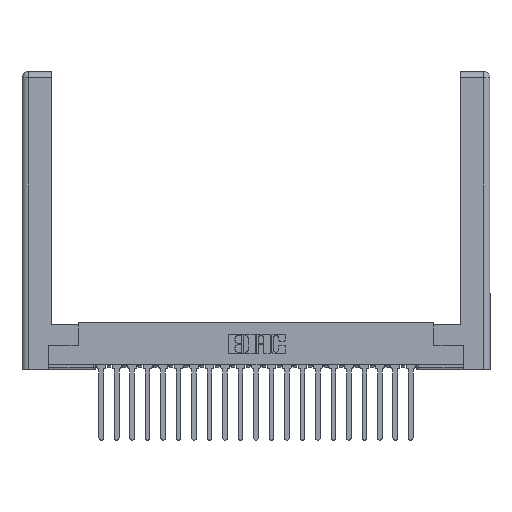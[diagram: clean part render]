
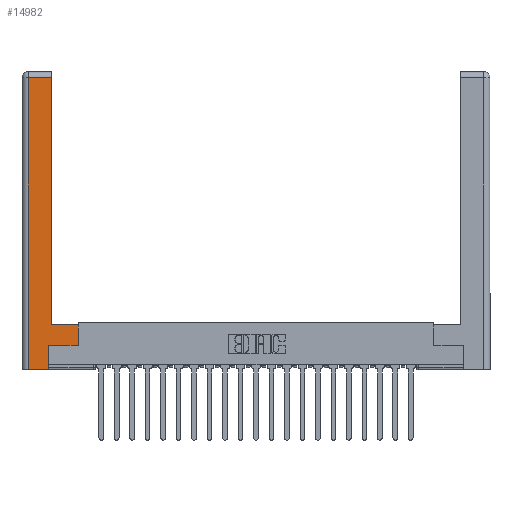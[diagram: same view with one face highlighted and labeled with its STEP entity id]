
A CAD part, top view. The second image highlights one B-rep face of the part: STEP entity #14982.
In plain terms, the highlighted planar face has unit normal (0, 0, 1).
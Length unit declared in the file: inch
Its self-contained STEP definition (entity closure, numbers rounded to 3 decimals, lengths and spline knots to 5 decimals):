
#617 = CARTESIAN_POINT ( 'NONE',  ( 0.0615, 2.94, 0. ) ) ;
#858 = PLANE ( 'NONE',  #6192 ) ;
#1038 = DIRECTION ( 'NONE',  ( 0., 1., 0. ) ) ;
#1102 = VERTEX_POINT ( 'NONE', #7507 ) ;
#2020 = CARTESIAN_POINT ( 'NONE',  ( 0.0615, 2.94, 0. ) ) ;
#2533 = VECTOR ( 'NONE', #12860, 39.37008 ) ;
#2578 = DIRECTION ( 'NONE',  ( 0., 1., 0. ) ) ;
#2597 = CARTESIAN_POINT ( 'NONE',  ( 0., 0., 0. ) ) ;
#2929 = FACE_OUTER_BOUND ( 'NONE', #4494, .T. ) ;
#3064 = EDGE_CURVE ( 'NONE', #12046, #16236, #20750, .T. ) ;
#3332 = EDGE_CURVE ( 'NONE', #23174, #12046, #17524, .T. ) ;
#3719 = ORIENTED_EDGE ( 'NONE', *, *, #6815, .T. ) ;
#3980 = ORIENTED_EDGE ( 'NONE', *, *, #19150, .T. ) ;
#4494 = EDGE_LOOP ( 'NONE', ( #23071, #3719, #3980, #4528, #10552, #19849, #20191, #16464 ) ) ;
#4528 = ORIENTED_EDGE ( 'NONE', *, *, #7918, .T. ) ;
#6113 = CARTESIAN_POINT ( 'NONE',  ( 0.295, 3., 0. ) ) ;
#6173 = LINE ( 'NONE', #617, #2533 ) ;
#6192 = AXIS2_PLACEMENT_3D ( 'NONE', #2597, #22149, #8065 ) ;
#6324 = CARTESIAN_POINT ( 'NONE',  ( 0.565, 0.245, 0. ) ) ;
#6553 = DIRECTION ( 'NONE',  ( 0., -1., 0. ) ) ;
#6815 = EDGE_CURVE ( 'NONE', #16236, #9266, #6173, .T. ) ;
#7507 = CARTESIAN_POINT ( 'NONE',  ( 0.265, 0., 0. ) ) ;
#7607 = VERTEX_POINT ( 'NONE', #6324 ) ;
#7918 = EDGE_CURVE ( 'NONE', #12849, #1102, #9459, .T. ) ;
#8065 = DIRECTION ( 'NONE',  ( -1., 0., 0. ) ) ;
#9266 = VERTEX_POINT ( 'NONE', #2020 ) ;
#9459 = LINE ( 'NONE', #15742, #12246 ) ;
#10511 = VECTOR ( 'NONE', #20896, 39.37008 ) ;
#10552 = ORIENTED_EDGE ( 'NONE', *, *, #19860, .T. ) ;
#11117 = DIRECTION ( 'NONE',  ( 0., 1., 0. ) ) ;
#11160 = EDGE_CURVE ( 'NONE', #7607, #23174, #21858, .T. ) ;
#11485 = VECTOR ( 'NONE', #1038, 39.37008 ) ;
#11532 = VECTOR ( 'NONE', #11117, 39.37008 ) ;
#11841 = LINE ( 'NONE', #11936, #18846 ) ;
#11936 = CARTESIAN_POINT ( 'NONE',  ( 0.0615, 0., 0. ) ) ;
#12046 = VERTEX_POINT ( 'NONE', #19767 ) ;
#12246 = VECTOR ( 'NONE', #12384, 39.37008 ) ;
#12384 = DIRECTION ( 'NONE',  ( 1., 0., 0. ) ) ;
#12849 = VERTEX_POINT ( 'NONE', #20310 ) ;
#12860 = DIRECTION ( 'NONE',  ( -1., 0., 0. ) ) ;
#13403 = VERTEX_POINT ( 'NONE', #16669 ) ;
#14428 = VECTOR ( 'NONE', #14737, 39.37008 ) ;
#14615 = LINE ( 'NONE', #17183, #18270 ) ;
#14737 = DIRECTION ( 'NONE',  ( 1., 0., 0. ) ) ;
#14982 = ADVANCED_FACE ( 'NONE', ( #2929 ), #858, .F. ) ;
#15058 = CARTESIAN_POINT ( 'NONE',  ( 0.295, 2.94, 0. ) ) ;
#15742 = CARTESIAN_POINT ( 'NONE',  ( 0.265, 0., 0. ) ) ;
#16236 = VERTEX_POINT ( 'NONE', #15058 ) ;
#16464 = ORIENTED_EDGE ( 'NONE', *, *, #3332, .T. ) ;
#16669 = CARTESIAN_POINT ( 'NONE',  ( 0.265, 0.245, 0. ) ) ;
#17183 = CARTESIAN_POINT ( 'NONE',  ( 0.265, 0.245, 0. ) ) ;
#17524 = LINE ( 'NONE', #22621, #10511 ) ;
#18270 = VECTOR ( 'NONE', #2578, 39.37008 ) ;
#18422 = CARTESIAN_POINT ( 'NONE',  ( 0.565, 0.245, 0. ) ) ;
#18846 = VECTOR ( 'NONE', #6553, 39.37008 ) ;
#19150 = EDGE_CURVE ( 'NONE', #9266, #12849, #11841, .T. ) ;
#19767 = CARTESIAN_POINT ( 'NONE',  ( 0.295, 0.45, 0. ) ) ;
#19849 = ORIENTED_EDGE ( 'NONE', *, *, #22344, .T. ) ;
#19860 = EDGE_CURVE ( 'NONE', #1102, #13403, #14615, .T. ) ;
#20191 = ORIENTED_EDGE ( 'NONE', *, *, #11160, .T. ) ;
#20310 = CARTESIAN_POINT ( 'NONE',  ( 0.0615, 0., 0. ) ) ;
#20653 = LINE ( 'NONE', #18422, #14428 ) ;
#20750 = LINE ( 'NONE', #6113, #11532 ) ;
#20896 = DIRECTION ( 'NONE',  ( -1., 0., 0. ) ) ;
#21858 = LINE ( 'NONE', #22268, #11485 ) ;
#22149 = DIRECTION ( 'NONE',  ( 0., 0., -1. ) ) ;
#22268 = CARTESIAN_POINT ( 'NONE',  ( 0.565, 0.45, 0. ) ) ;
#22344 = EDGE_CURVE ( 'NONE', #13403, #7607, #20653, .T. ) ;
#22621 = CARTESIAN_POINT ( 'NONE',  ( 0.295, 0.45, 0. ) ) ;
#22971 = CARTESIAN_POINT ( 'NONE',  ( 0.565, 0.45, 0. ) ) ;
#23071 = ORIENTED_EDGE ( 'NONE', *, *, #3064, .T. ) ;
#23174 = VERTEX_POINT ( 'NONE', #22971 ) ;
